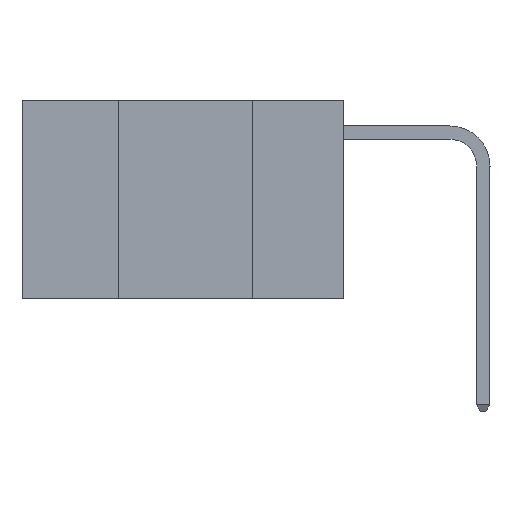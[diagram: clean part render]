
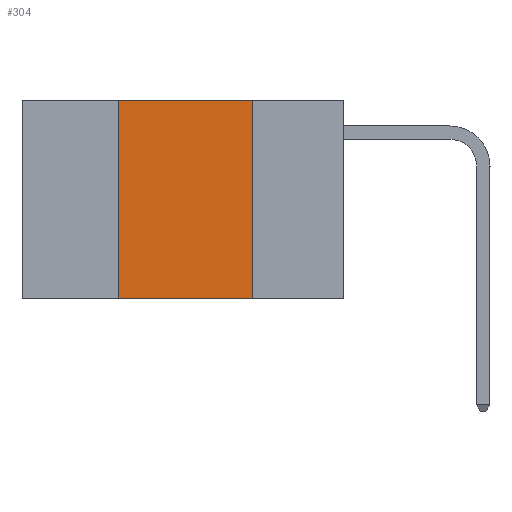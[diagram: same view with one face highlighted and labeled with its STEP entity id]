
A CAD part, left-side view. The second image highlights one B-rep face of the part: STEP entity #304.
In plain terms, the highlighted planar face has unit normal (-1, 0, 0).
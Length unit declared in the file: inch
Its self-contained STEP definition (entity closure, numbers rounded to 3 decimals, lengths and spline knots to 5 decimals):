
#304 = ADVANCED_FACE ( 'NONE', ( #488 ), #473, .F. ) ;
#473 = PLANE ( 'NONE',  #1379 ) ;
#488 = FACE_OUTER_BOUND ( 'NONE', #12028, .T. ) ;
#565 = EDGE_CURVE ( 'NONE', #11395, #9924, #10147, .T. ) ;
#1379 = AXIS2_PLACEMENT_3D ( 'NONE', #7985, #10526, #11097 ) ;
#1824 = CARTESIAN_POINT ( 'NONE',  ( 0., 0.42, 0. ) ) ;
#1955 = VERTEX_POINT ( 'NONE', #4796 ) ;
#2129 = VERTEX_POINT ( 'NONE', #1824 ) ;
#2566 = LINE ( 'NONE', #8800, #9766 ) ;
#2771 = CARTESIAN_POINT ( 'NONE',  ( 0., 0.17, 0. ) ) ;
#2783 = LINE ( 'NONE', #9003, #9975 ) ;
#3164 = DIRECTION ( 'NONE',  ( 0., -1., 0. ) ) ;
#3446 = CARTESIAN_POINT ( 'NONE',  ( 0., 0.17, -0.37 ) ) ;
#4295 = LINE ( 'NONE', #5850, #11330 ) ;
#4377 = DIRECTION ( 'NONE',  ( 0., 0., -1. ) ) ;
#4796 = CARTESIAN_POINT ( 'NONE',  ( 0., 0.42, -0.37 ) ) ;
#4863 = ORIENTED_EDGE ( 'NONE', *, *, #6735, .F. ) ;
#5850 = CARTESIAN_POINT ( 'NONE',  ( 0., 0.42, 0. ) ) ;
#6735 = EDGE_CURVE ( 'NONE', #1955, #2129, #4295, .T. ) ;
#7550 = EDGE_CURVE ( 'NONE', #2129, #11395, #2566, .T. ) ;
#7985 = CARTESIAN_POINT ( 'NONE',  ( 0., 0.6, 0. ) ) ;
#8013 = VECTOR ( 'NONE', #4377, 39.37008 ) ;
#8655 = ORIENTED_EDGE ( 'NONE', *, *, #565, .F. ) ;
#8800 = CARTESIAN_POINT ( 'NONE',  ( 0., 0.6, 0. ) ) ;
#9003 = CARTESIAN_POINT ( 'NONE',  ( 0., 0.6, -0.37 ) ) ;
#9039 = DIRECTION ( 'NONE',  ( 0., -1., 0. ) ) ;
#9477 = ORIENTED_EDGE ( 'NONE', *, *, #10458, .T. ) ;
#9489 = CARTESIAN_POINT ( 'NONE',  ( 0., 0.17, 0. ) ) ;
#9766 = VECTOR ( 'NONE', #3164, 39.37008 ) ;
#9924 = VERTEX_POINT ( 'NONE', #3446 ) ;
#9975 = VECTOR ( 'NONE', #9039, 39.37008 ) ;
#10147 = LINE ( 'NONE', #2771, #8013 ) ;
#10386 = DIRECTION ( 'NONE',  ( 0., 0., 1. ) ) ;
#10458 = EDGE_CURVE ( 'NONE', #1955, #9924, #2783, .T. ) ;
#10526 = DIRECTION ( 'NONE',  ( 1., 0., 0. ) ) ;
#11065 = ORIENTED_EDGE ( 'NONE', *, *, #7550, .F. ) ;
#11097 = DIRECTION ( 'NONE',  ( 0., 0., -1. ) ) ;
#11330 = VECTOR ( 'NONE', #10386, 39.37008 ) ;
#11395 = VERTEX_POINT ( 'NONE', #9489 ) ;
#12028 = EDGE_LOOP ( 'NONE', ( #8655, #11065, #4863, #9477 ) ) ;
